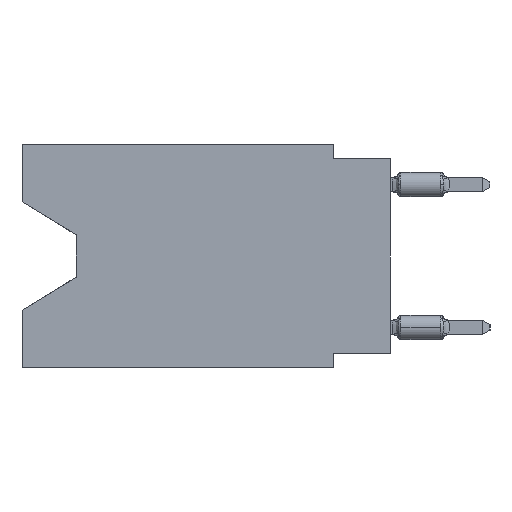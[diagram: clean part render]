
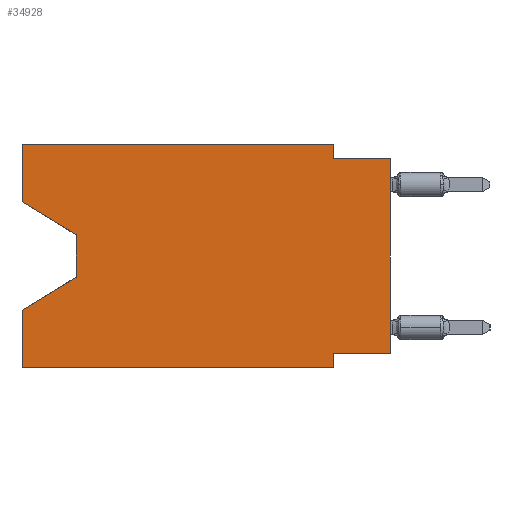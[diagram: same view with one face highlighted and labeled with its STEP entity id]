
A CAD part, left-side view. The second image highlights one B-rep face of the part: STEP entity #34928.
In plain terms, the highlighted planar face has unit normal (-1, 0, 0).
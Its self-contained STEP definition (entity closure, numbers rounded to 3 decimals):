
#817 = VECTOR ( 'NONE', #27291, 1000. ) ;
#2428 = VERTEX_POINT ( 'NONE', #19432 ) ;
#2607 = DIRECTION ( 'NONE',  ( 0., 0., -1. ) ) ;
#2625 = VECTOR ( 'NONE', #11628, 1000. ) ;
#2738 = CARTESIAN_POINT ( 'NONE',  ( 0., 13.97, -4.013 ) ) ;
#3009 = DIRECTION ( 'NONE',  ( 0., 0., -1. ) ) ;
#4033 = LINE ( 'NONE', #18922, #26273 ) ;
#4613 = EDGE_CURVE ( 'NONE', #16077, #39668, #26402, .T. ) ;
#4987 = VERTEX_POINT ( 'NONE', #16334 ) ;
#5680 = VECTOR ( 'NONE', #24177, 1000. ) ;
#5784 = LINE ( 'NONE', #16997, #45129 ) ;
#7218 = CARTESIAN_POINT ( 'NONE',  ( 0., 0., -0.635 ) ) ;
#8530 = CARTESIAN_POINT ( 'NONE',  ( 0., 2.54, 0. ) ) ;
#9106 = EDGE_CURVE ( 'NONE', #22073, #13985, #5784, .T. ) ;
#9467 = ORIENTED_EDGE ( 'NONE', *, *, #9897, .F. ) ;
#9897 = EDGE_CURVE ( 'NONE', #39668, #16101, #12435, .T. ) ;
#10114 = CARTESIAN_POINT ( 'NONE',  ( 0., 0., -0.635 ) ) ;
#10552 = CARTESIAN_POINT ( 'NONE',  ( 0., 0., -9.271 ) ) ;
#10912 = VERTEX_POINT ( 'NONE', #14960 ) ;
#11196 = LINE ( 'NONE', #29248, #23455 ) ;
#11259 = LINE ( 'NONE', #10552, #23526 ) ;
#11628 = DIRECTION ( 'NONE',  ( 0., 0., 1. ) ) ;
#11698 = ORIENTED_EDGE ( 'NONE', *, *, #16226, .F. ) ;
#12435 = LINE ( 'NONE', #31212, #817 ) ;
#13246 = CARTESIAN_POINT ( 'NONE',  ( 0., 13.97, -5.893 ) ) ;
#13985 = VERTEX_POINT ( 'NONE', #13246 ) ;
#13986 = EDGE_CURVE ( 'NONE', #13985, #2428, #24927, .T. ) ;
#14279 = AXIS2_PLACEMENT_3D ( 'NONE', #32538, #44703, #3009 ) ;
#14480 = ORIENTED_EDGE ( 'NONE', *, *, #13986, .T. ) ;
#14871 = VECTOR ( 'NONE', #24967, 1000. ) ;
#14960 = CARTESIAN_POINT ( 'NONE',  ( 0., 16.383, -2.546 ) ) ;
#15676 = LINE ( 'NONE', #35875, #5680 ) ;
#16045 = CARTESIAN_POINT ( 'NONE',  ( 0., 16.383, 0. ) ) ;
#16077 = VERTEX_POINT ( 'NONE', #33598 ) ;
#16101 = VERTEX_POINT ( 'NONE', #40012 ) ;
#16226 = EDGE_CURVE ( 'NONE', #10912, #16077, #30671, .T. ) ;
#16334 = CARTESIAN_POINT ( 'NONE',  ( 0., 2.54, -9.906 ) ) ;
#16418 = VERTEX_POINT ( 'NONE', #7218 ) ;
#16921 = DIRECTION ( 'NONE',  ( 0., 0.855, -0.519 ) ) ;
#16997 = CARTESIAN_POINT ( 'NONE',  ( 0., 13.97, -4.013 ) ) ;
#18477 = LINE ( 'NONE', #26255, #2625 ) ;
#18922 = CARTESIAN_POINT ( 'NONE',  ( 0., 16.383, -2.546 ) ) ;
#19432 = CARTESIAN_POINT ( 'NONE',  ( 0., 16.383, -7.36 ) ) ;
#20111 = EDGE_CURVE ( 'NONE', #10912, #22073, #4033, .T. ) ;
#20188 = CARTESIAN_POINT ( 'NONE',  ( 0., 0., -9.271 ) ) ;
#20755 = EDGE_CURVE ( 'NONE', #31361, #4987, #15676, .T. ) ;
#21780 = PLANE ( 'NONE',  #14279 ) ;
#22073 = VERTEX_POINT ( 'NONE', #2738 ) ;
#22102 = ORIENTED_EDGE ( 'NONE', *, *, #25952, .F. ) ;
#22154 = EDGE_CURVE ( 'NONE', #42999, #27929, #11259, .T. ) ;
#22872 = DIRECTION ( 'NONE',  ( 0., 0., 1. ) ) ;
#23455 = VECTOR ( 'NONE', #44122, 1000. ) ;
#23526 = VECTOR ( 'NONE', #40758, 1000. ) ;
#24086 = CARTESIAN_POINT ( 'NONE',  ( 0., 16.383, -9.906 ) ) ;
#24177 = DIRECTION ( 'NONE',  ( 0., -1., 0. ) ) ;
#24828 = DIRECTION ( 'NONE',  ( 0., 0., 1. ) ) ;
#24927 = LINE ( 'NONE', #39803, #46929 ) ;
#24967 = DIRECTION ( 'NONE',  ( 0., -1., 0. ) ) ;
#25293 = VECTOR ( 'NONE', #22872, 1000. ) ;
#25835 = ORIENTED_EDGE ( 'NONE', *, *, #38169, .F. ) ;
#25952 = EDGE_CURVE ( 'NONE', #16101, #16418, #28881, .T. ) ;
#26255 = CARTESIAN_POINT ( 'NONE',  ( 0., 16.383, 0. ) ) ;
#26273 = VECTOR ( 'NONE', #29184, 1000. ) ;
#26402 = LINE ( 'NONE', #41276, #36175 ) ;
#27099 = ORIENTED_EDGE ( 'NONE', *, *, #9106, .T. ) ;
#27291 = DIRECTION ( 'NONE',  ( 0., 0., -1. ) ) ;
#27805 = ORIENTED_EDGE ( 'NONE', *, *, #30417, .F. ) ;
#27929 = VERTEX_POINT ( 'NONE', #37638 ) ;
#28252 = VECTOR ( 'NONE', #24828, 1000. ) ;
#28881 = LINE ( 'NONE', #10114, #14871 ) ;
#29184 = DIRECTION ( 'NONE',  ( 0., -0.855, -0.519 ) ) ;
#29248 = CARTESIAN_POINT ( 'NONE',  ( 0., 2.54, -9.906 ) ) ;
#30189 = ORIENTED_EDGE ( 'NONE', *, *, #4613, .F. ) ;
#30417 = EDGE_CURVE ( 'NONE', #31361, #2428, #18477, .T. ) ;
#30450 = EDGE_LOOP ( 'NONE', ( #31688, #27099, #14480, #27805, #37978, #25835, #31321, #42410, #22102, #9467, #30189, #11698 ) ) ;
#30671 = LINE ( 'NONE', #16045, #25293 ) ;
#31212 = CARTESIAN_POINT ( 'NONE',  ( 0., 2.54, 0. ) ) ;
#31321 = ORIENTED_EDGE ( 'NONE', *, *, #22154, .F. ) ;
#31361 = VERTEX_POINT ( 'NONE', #24086 ) ;
#31688 = ORIENTED_EDGE ( 'NONE', *, *, #20111, .T. ) ;
#32538 = CARTESIAN_POINT ( 'NONE',  ( 0., 16.383, 0. ) ) ;
#32782 = DIRECTION ( 'NONE',  ( 0., -1., 0. ) ) ;
#33598 = CARTESIAN_POINT ( 'NONE',  ( 0., 16.383, 0. ) ) ;
#34928 = ADVANCED_FACE ( 'NONE', ( #36667 ), #21780, .F. ) ;
#35875 = CARTESIAN_POINT ( 'NONE',  ( 0., 16.383, -9.906 ) ) ;
#36175 = VECTOR ( 'NONE', #32782, 1000. ) ;
#36667 = FACE_OUTER_BOUND ( 'NONE', #30450, .T. ) ;
#37638 = CARTESIAN_POINT ( 'NONE',  ( 0., 2.54, -9.271 ) ) ;
#37978 = ORIENTED_EDGE ( 'NONE', *, *, #20755, .T. ) ;
#38169 = EDGE_CURVE ( 'NONE', #27929, #4987, #11196, .T. ) ;
#39471 = CARTESIAN_POINT ( 'NONE',  ( 0., 0., 0. ) ) ;
#39668 = VERTEX_POINT ( 'NONE', #8530 ) ;
#39803 = CARTESIAN_POINT ( 'NONE',  ( 0., 13.97, -5.893 ) ) ;
#39851 = EDGE_CURVE ( 'NONE', #42999, #16418, #44118, .T. ) ;
#40012 = CARTESIAN_POINT ( 'NONE',  ( 0., 2.54, -0.635 ) ) ;
#40758 = DIRECTION ( 'NONE',  ( 0., 1., 0. ) ) ;
#41276 = CARTESIAN_POINT ( 'NONE',  ( 0., 16.383, 0. ) ) ;
#42410 = ORIENTED_EDGE ( 'NONE', *, *, #39851, .T. ) ;
#42999 = VERTEX_POINT ( 'NONE', #20188 ) ;
#44118 = LINE ( 'NONE', #39471, #28252 ) ;
#44122 = DIRECTION ( 'NONE',  ( 0., 0., -1. ) ) ;
#44703 = DIRECTION ( 'NONE',  ( 1., 0., 0. ) ) ;
#45129 = VECTOR ( 'NONE', #2607, 1000. ) ;
#46929 = VECTOR ( 'NONE', #16921, 1000. ) ;
